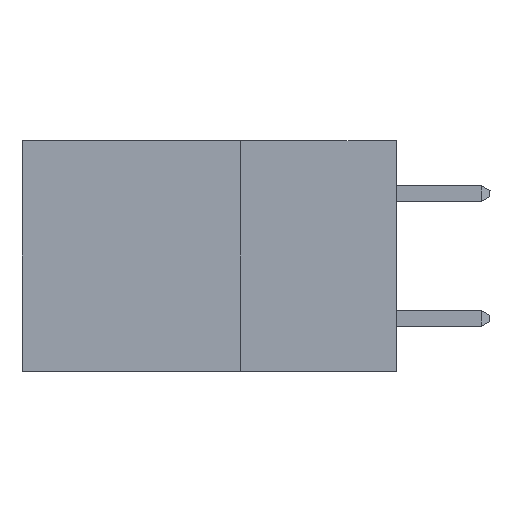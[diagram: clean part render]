
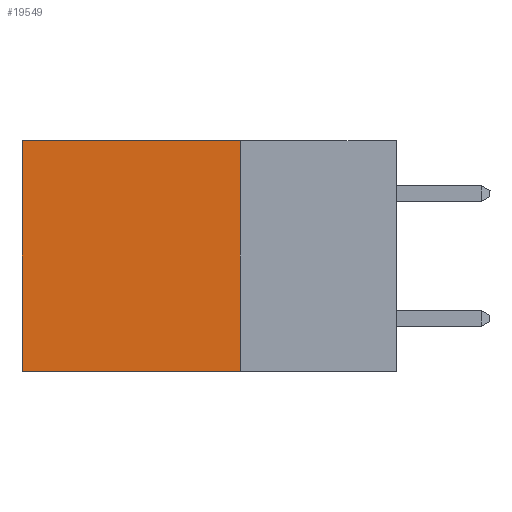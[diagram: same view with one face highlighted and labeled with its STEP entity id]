
A CAD part, left-side view. The second image highlights one B-rep face of the part: STEP entity #19549.
In plain terms, the highlighted planar face has unit normal (-1, 0, 0).
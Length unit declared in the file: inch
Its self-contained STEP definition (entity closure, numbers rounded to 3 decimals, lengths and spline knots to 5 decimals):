
#523 = LINE ( 'NONE', #2379, #12542 ) ;
#536 = VECTOR ( 'NONE', #14380, 39.37008 ) ;
#655 = VECTOR ( 'NONE', #9514, 39.37008 ) ;
#2379 = CARTESIAN_POINT ( 'NONE',  ( 0.298, 0.25, 0. ) ) ;
#3908 = EDGE_LOOP ( 'NONE', ( #23715, #8345, #7302, #27731 ) ) ;
#4802 = DIRECTION ( 'NONE',  ( 0., 0., -1. ) ) ;
#5374 = FACE_OUTER_BOUND ( 'NONE', #3908, .T. ) ;
#6051 = CARTESIAN_POINT ( 'NONE',  ( 0.298, 0.25, 0. ) ) ;
#6671 = LINE ( 'NONE', #16147, #18607 ) ;
#7302 = ORIENTED_EDGE ( 'NONE', *, *, #27969, .F. ) ;
#7757 = LINE ( 'NONE', #18944, #655 ) ;
#8345 = ORIENTED_EDGE ( 'NONE', *, *, #23110, .F. ) ;
#9514 = DIRECTION ( 'NONE',  ( 0., 1., 0. ) ) ;
#11195 = EDGE_CURVE ( 'NONE', #24031, #21412, #6671, .T. ) ;
#11998 = CARTESIAN_POINT ( 'NONE',  ( 0.298, 0.6, 0. ) ) ;
#12542 = VECTOR ( 'NONE', #4802, 39.37008 ) ;
#13297 = LINE ( 'NONE', #11998, #536 ) ;
#14380 = DIRECTION ( 'NONE',  ( 0., 0., -1. ) ) ;
#14584 = DIRECTION ( 'NONE',  ( 0., 0., -1. ) ) ;
#16147 = CARTESIAN_POINT ( 'NONE',  ( 0.298, 0.25, 0. ) ) ;
#17413 = CARTESIAN_POINT ( 'NONE',  ( 0.298, 0.25, -0.37 ) ) ;
#18354 = AXIS2_PLACEMENT_3D ( 'NONE', #26255, #28606, #14584 ) ;
#18500 = DIRECTION ( 'NONE',  ( 0., 1., 0. ) ) ;
#18607 = VECTOR ( 'NONE', #18500, 39.37008 ) ;
#18944 = CARTESIAN_POINT ( 'NONE',  ( 0.298, 0.25, -0.37 ) ) ;
#19468 = EDGE_CURVE ( 'NONE', #21412, #20085, #13297, .T. ) ;
#19549 = ADVANCED_FACE ( 'NONE', ( #5374 ), #23866, .F. ) ;
#20085 = VERTEX_POINT ( 'NONE', #28267 ) ;
#21412 = VERTEX_POINT ( 'NONE', #26197 ) ;
#23110 = EDGE_CURVE ( 'NONE', #26481, #20085, #7757, .T. ) ;
#23715 = ORIENTED_EDGE ( 'NONE', *, *, #19468, .T. ) ;
#23866 = PLANE ( 'NONE',  #18354 ) ;
#24031 = VERTEX_POINT ( 'NONE', #6051 ) ;
#26197 = CARTESIAN_POINT ( 'NONE',  ( 0.298, 0.6, 0. ) ) ;
#26255 = CARTESIAN_POINT ( 'NONE',  ( 0.298, 0.25, 0. ) ) ;
#26481 = VERTEX_POINT ( 'NONE', #17413 ) ;
#27731 = ORIENTED_EDGE ( 'NONE', *, *, #11195, .T. ) ;
#27969 = EDGE_CURVE ( 'NONE', #24031, #26481, #523, .T. ) ;
#28267 = CARTESIAN_POINT ( 'NONE',  ( 0.298, 0.6, -0.37 ) ) ;
#28606 = DIRECTION ( 'NONE',  ( 1., 0., 0. ) ) ;
